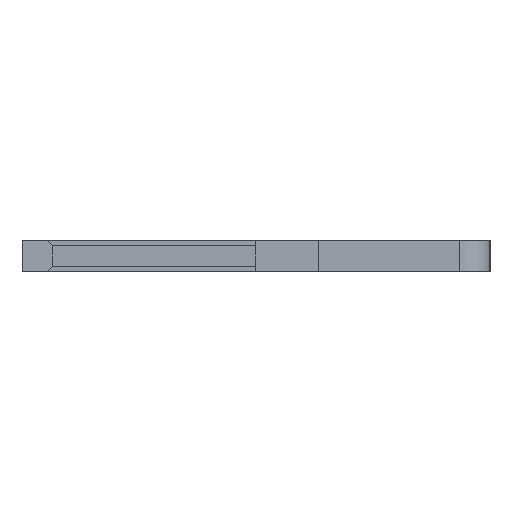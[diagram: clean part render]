
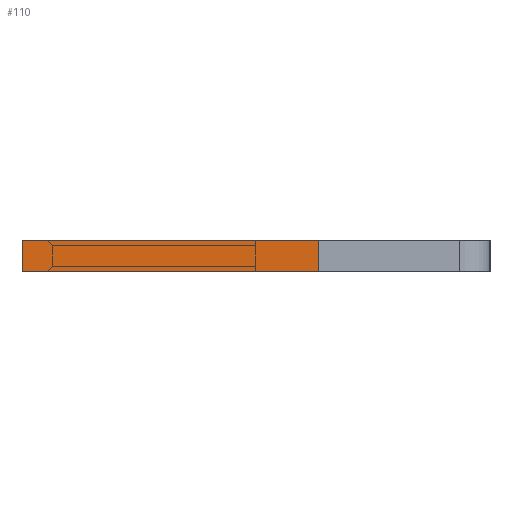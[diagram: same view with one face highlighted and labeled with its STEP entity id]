
A CAD part, left-side view. The second image highlights one B-rep face of the part: STEP entity #110.
In plain terms, the highlighted face is planar.
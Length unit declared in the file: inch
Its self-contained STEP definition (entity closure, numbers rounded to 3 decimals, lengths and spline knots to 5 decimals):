
#105 = DIRECTION ( 'NONE',  ( 0., 0., 1. ) ) ;
#106 = CARTESIAN_POINT ( 'NONE',  ( -0.01, -0.04, -0.04 ) ) ;
#110 = ADVANCED_FACE ( 'NONE', ( #2368 ), #2656, .F. ) ;
#133 = VECTOR ( 'NONE', #1690, 39.37008 ) ;
#305 = LINE ( 'NONE', #1535, #3522 ) ;
#367 = ORIENTED_EDGE ( 'NONE', *, *, #3293, .F. ) ;
#405 = VECTOR ( 'NONE', #1838, 39.37008 ) ;
#519 = CARTESIAN_POINT ( 'NONE',  ( 0.01, 0.15, -0.04 ) ) ;
#570 = EDGE_CURVE ( 'NONE', #2996, #2157, #2453, .T. ) ;
#996 = ORIENTED_EDGE ( 'NONE', *, *, #3005, .F. ) ;
#1065 = LINE ( 'NONE', #2333, #133 ) ;
#1234 = EDGE_CURVE ( 'NONE', #2703, #2996, #1065, .T. ) ;
#1252 = LINE ( 'NONE', #2159, #3320 ) ;
#1535 = CARTESIAN_POINT ( 'NONE',  ( 0.01, 0.15, -0.04 ) ) ;
#1564 = DIRECTION ( 'NONE',  ( 0., 1., 0. ) ) ;
#1690 = DIRECTION ( 'NONE',  ( -1., 0., 0. ) ) ;
#1714 = EDGE_LOOP ( 'NONE', ( #2778, #996, #367, #2244 ) ) ;
#1838 = DIRECTION ( 'NONE',  ( 0., 1., 0. ) ) ;
#1924 = VERTEX_POINT ( 'NONE', #519 ) ;
#2112 = DIRECTION ( 'NONE',  ( 1., 0., 0. ) ) ;
#2157 = VERTEX_POINT ( 'NONE', #2238 ) ;
#2159 = CARTESIAN_POINT ( 'NONE',  ( 0.01, 0.15, -0.04 ) ) ;
#2238 = CARTESIAN_POINT ( 'NONE',  ( -0.01, 0.15, -0.04 ) ) ;
#2244 = ORIENTED_EDGE ( 'NONE', *, *, #1234, .T. ) ;
#2333 = CARTESIAN_POINT ( 'NONE',  ( 0.01, -0.04, -0.04 ) ) ;
#2368 = FACE_OUTER_BOUND ( 'NONE', #1714, .T. ) ;
#2453 = LINE ( 'NONE', #2690, #405 ) ;
#2656 = PLANE ( 'NONE',  #3051 ) ;
#2690 = CARTESIAN_POINT ( 'NONE',  ( -0.01, 0.15, -0.04 ) ) ;
#2703 = VERTEX_POINT ( 'NONE', #3473 ) ;
#2778 = ORIENTED_EDGE ( 'NONE', *, *, #570, .T. ) ;
#2996 = VERTEX_POINT ( 'NONE', #106 ) ;
#3005 = EDGE_CURVE ( 'NONE', #1924, #2157, #305, .T. ) ;
#3051 = AXIS2_PLACEMENT_3D ( 'NONE', #3223, #105, #2112 ) ;
#3223 = CARTESIAN_POINT ( 'NONE',  ( 0.01, 0.15, -0.04 ) ) ;
#3293 = EDGE_CURVE ( 'NONE', #2703, #1924, #1252, .T. ) ;
#3320 = VECTOR ( 'NONE', #1564, 39.37008 ) ;
#3473 = CARTESIAN_POINT ( 'NONE',  ( 0.01, -0.04, -0.04 ) ) ;
#3495 = DIRECTION ( 'NONE',  ( -1., 0., 0. ) ) ;
#3522 = VECTOR ( 'NONE', #3495, 39.37008 ) ;
